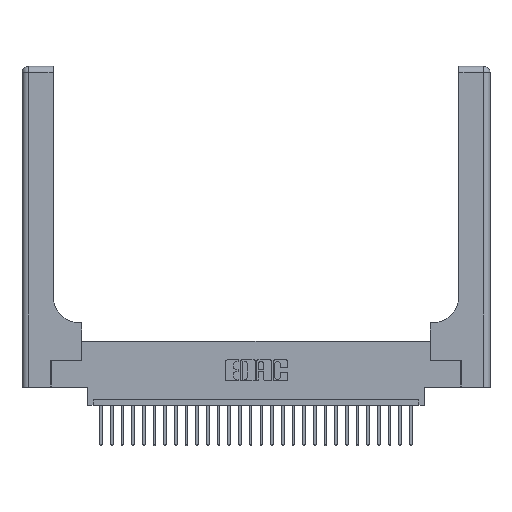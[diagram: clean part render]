
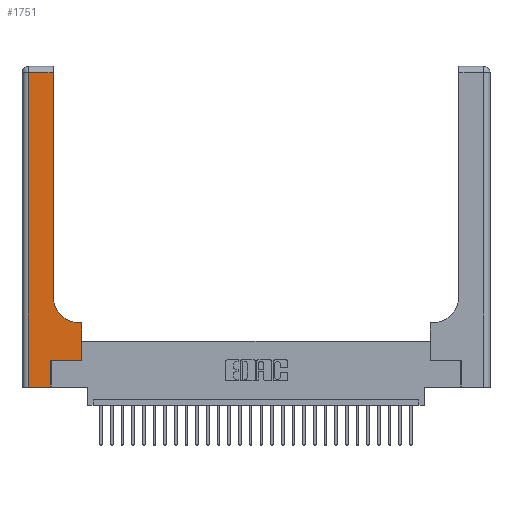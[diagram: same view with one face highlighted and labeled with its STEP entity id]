
A CAD part, top view. The second image highlights one B-rep face of the part: STEP entity #1751.
In plain terms, the highlighted planar face has unit normal (0, 0, 1).
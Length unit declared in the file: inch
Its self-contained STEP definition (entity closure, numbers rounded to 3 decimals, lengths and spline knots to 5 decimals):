
#253 = VERTEX_POINT ( 'NONE', #27643 ) ;
#649 = CARTESIAN_POINT ( 'NONE',  ( 0., 2.94, 0.37 ) ) ;
#1087 = EDGE_CURVE ( 'NONE', #16476, #13917, #16705, .T. ) ;
#1197 = VECTOR ( 'NONE', #17520, 39.37008 ) ;
#1751 = ADVANCED_FACE ( 'NONE', ( #19785 ), #9833, .F. ) ;
#2019 = VERTEX_POINT ( 'NONE', #14833 ) ;
#3282 = LINE ( 'NONE', #649, #15383 ) ;
#3595 = DIRECTION ( 'NONE',  ( 0., 1., 0. ) ) ;
#3604 = CARTESIAN_POINT ( 'NONE',  ( 0.5585, 0.6, 0.37 ) ) ;
#3776 = EDGE_CURVE ( 'NONE', #13551, #11698, #13655, .T. ) ;
#4375 = VECTOR ( 'NONE', #20358, 39.37008 ) ;
#4435 = CARTESIAN_POINT ( 'NONE',  ( 0.2915, 3., 0.37 ) ) ;
#5557 = CARTESIAN_POINT ( 'NONE',  ( 0.5415, 0.6, 0.37 ) ) ;
#5573 = EDGE_LOOP ( 'NONE', ( #26866, #15732, #16653, #22901, #23521, #21104, #14409, #6882, #28509 ) ) ;
#5698 = VECTOR ( 'NONE', #10347, 39.37008 ) ;
#6201 = EDGE_CURVE ( 'NONE', #28600, #13551, #8506, .T. ) ;
#6623 = VECTOR ( 'NONE', #7672, 39.37008 ) ;
#6882 = ORIENTED_EDGE ( 'NONE', *, *, #21151, .T. ) ;
#6974 = CARTESIAN_POINT ( 'NONE',  ( 0.2915, 0.6, 0.37 ) ) ;
#7672 = DIRECTION ( 'NONE',  ( 0., -1., 0. ) ) ;
#8349 = CARTESIAN_POINT ( 'NONE',  ( 0.269, 0., 0.37 ) ) ;
#8465 = VECTOR ( 'NONE', #18515, 39.37008 ) ;
#8506 = CIRCLE ( 'NONE', #21109, 0.25 ) ;
#8883 = CARTESIAN_POINT ( 'NONE',  ( 0.06, 3., 0.37 ) ) ;
#9267 = VERTEX_POINT ( 'NONE', #3604 ) ;
#9466 = CARTESIAN_POINT ( 'NONE',  ( 0.5415, 0.85, 0.37 ) ) ;
#9833 = PLANE ( 'NONE',  #11271 ) ;
#10347 = DIRECTION ( 'NONE',  ( 1., 0., 0. ) ) ;
#10792 = CARTESIAN_POINT ( 'NONE',  ( 0.269, 0.25, 0.37 ) ) ;
#10829 = CARTESIAN_POINT ( 'NONE',  ( 0.2915, 2.94, 0.37 ) ) ;
#10976 = VECTOR ( 'NONE', #3595, 39.37008 ) ;
#11271 = AXIS2_PLACEMENT_3D ( 'NONE', #28270, #21411, #12046 ) ;
#11698 = VERTEX_POINT ( 'NONE', #10829 ) ;
#11744 = LINE ( 'NONE', #24257, #5698 ) ;
#12046 = DIRECTION ( 'NONE',  ( -1., 0., 0. ) ) ;
#12608 = CARTESIAN_POINT ( 'NONE',  ( 0.5585, 0.25, 0.37 ) ) ;
#12830 = CARTESIAN_POINT ( 'NONE',  ( 0.269, 0., 0.37 ) ) ;
#13551 = VERTEX_POINT ( 'NONE', #28117 ) ;
#13655 = LINE ( 'NONE', #4435, #4375 ) ;
#13917 = VERTEX_POINT ( 'NONE', #10792 ) ;
#14409 = ORIENTED_EDGE ( 'NONE', *, *, #28494, .T. ) ;
#14833 = CARTESIAN_POINT ( 'NONE',  ( 0.5585, 0.25, 0.37 ) ) ;
#15383 = VECTOR ( 'NONE', #16699, 39.37008 ) ;
#15575 = LINE ( 'NONE', #8883, #6623 ) ;
#15732 = ORIENTED_EDGE ( 'NONE', *, *, #24560, .T. ) ;
#16453 = DIRECTION ( 'NONE',  ( 1., 0., 0. ) ) ;
#16476 = VERTEX_POINT ( 'NONE', #12830 ) ;
#16653 = ORIENTED_EDGE ( 'NONE', *, *, #20856, .T. ) ;
#16699 = DIRECTION ( 'NONE',  ( -1., 0., 0. ) ) ;
#16705 = LINE ( 'NONE', #8349, #10976 ) ;
#17520 = DIRECTION ( 'NONE',  ( 1., 0., 0. ) ) ;
#18515 = DIRECTION ( 'NONE',  ( -1., 0., 0. ) ) ;
#18741 = LINE ( 'NONE', #12608, #24869 ) ;
#19311 = EDGE_CURVE ( 'NONE', #13917, #2019, #11744, .T. ) ;
#19785 = FACE_OUTER_BOUND ( 'NONE', #5573, .T. ) ;
#20358 = DIRECTION ( 'NONE',  ( 0., 1., 0. ) ) ;
#20856 = EDGE_CURVE ( 'NONE', #253, #28902, #15575, .T. ) ;
#20934 = DIRECTION ( 'NONE',  ( 0., 0., -1. ) ) ;
#21104 = ORIENTED_EDGE ( 'NONE', *, *, #19311, .T. ) ;
#21109 = AXIS2_PLACEMENT_3D ( 'NONE', #9466, #20934, #16453 ) ;
#21151 = EDGE_CURVE ( 'NONE', #9267, #28600, #22727, .T. ) ;
#21362 = CARTESIAN_POINT ( 'NONE',  ( 0., 0., 0.37 ) ) ;
#21411 = DIRECTION ( 'NONE',  ( 0., 0., -1. ) ) ;
#21892 = LINE ( 'NONE', #21362, #1197 ) ;
#22727 = LINE ( 'NONE', #6974, #8465 ) ;
#22901 = ORIENTED_EDGE ( 'NONE', *, *, #23030, .T. ) ;
#23030 = EDGE_CURVE ( 'NONE', #28902, #16476, #21892, .T. ) ;
#23521 = ORIENTED_EDGE ( 'NONE', *, *, #1087, .T. ) ;
#24024 = CARTESIAN_POINT ( 'NONE',  ( 0.06, 0., 0.37 ) ) ;
#24257 = CARTESIAN_POINT ( 'NONE',  ( 0.269, 0.25, 0.37 ) ) ;
#24560 = EDGE_CURVE ( 'NONE', #11698, #253, #3282, .T. ) ;
#24869 = VECTOR ( 'NONE', #26228, 39.37008 ) ;
#26228 = DIRECTION ( 'NONE',  ( 0., 1., 0. ) ) ;
#26866 = ORIENTED_EDGE ( 'NONE', *, *, #3776, .T. ) ;
#27643 = CARTESIAN_POINT ( 'NONE',  ( 0.06, 2.94, 0.37 ) ) ;
#28117 = CARTESIAN_POINT ( 'NONE',  ( 0.2915, 0.85, 0.37 ) ) ;
#28270 = CARTESIAN_POINT ( 'NONE',  ( 0., 3., 0.37 ) ) ;
#28494 = EDGE_CURVE ( 'NONE', #2019, #9267, #18741, .T. ) ;
#28509 = ORIENTED_EDGE ( 'NONE', *, *, #6201, .T. ) ;
#28600 = VERTEX_POINT ( 'NONE', #5557 ) ;
#28902 = VERTEX_POINT ( 'NONE', #24024 ) ;
